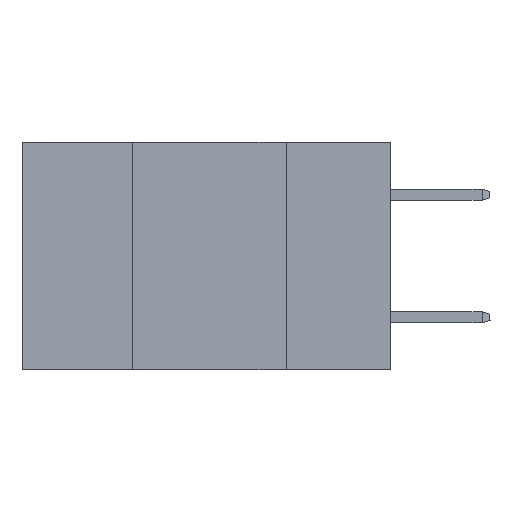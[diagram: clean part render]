
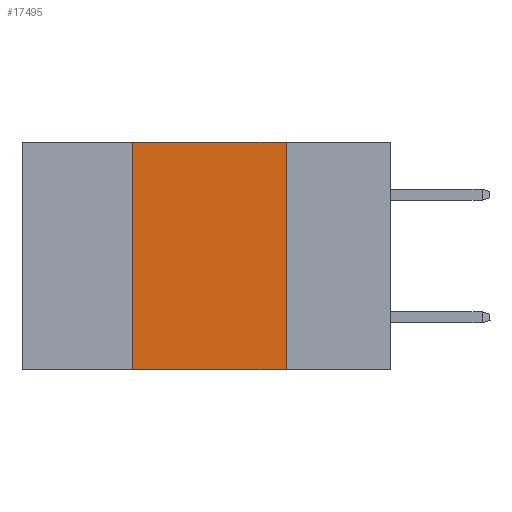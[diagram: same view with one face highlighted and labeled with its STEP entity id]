
A CAD part, left-side view. The second image highlights one B-rep face of the part: STEP entity #17495.
In plain terms, the highlighted planar face has unit normal (-1, 0, 0).
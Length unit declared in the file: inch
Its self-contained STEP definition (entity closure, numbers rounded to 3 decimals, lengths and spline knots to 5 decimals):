
#1050 = CARTESIAN_POINT ( 'NONE',  ( 0., 0.42, -0.37 ) ) ;
#1290 = CARTESIAN_POINT ( 'NONE',  ( 0., 0.17, 0. ) ) ;
#2728 = CARTESIAN_POINT ( 'NONE',  ( 0., 0.42, 0. ) ) ;
#3080 = EDGE_CURVE ( 'NONE', #3220, #10279, #19477, .T. ) ;
#3220 = VERTEX_POINT ( 'NONE', #1050 ) ;
#3921 = EDGE_LOOP ( 'NONE', ( #8095, #25872, #14075, #19346 ) ) ;
#4853 = PLANE ( 'NONE',  #8682 ) ;
#6683 = EDGE_CURVE ( 'NONE', #3220, #9972, #22991, .T. ) ;
#6812 = DIRECTION ( 'NONE',  ( 0., 0., -1. ) ) ;
#7413 = DIRECTION ( 'NONE',  ( 0., 0., -1. ) ) ;
#7713 = CARTESIAN_POINT ( 'NONE',  ( 0., 0.42, 0. ) ) ;
#8095 = ORIENTED_EDGE ( 'NONE', *, *, #16250, .F. ) ;
#8600 = VECTOR ( 'NONE', #19950, 39.37008 ) ;
#8682 = AXIS2_PLACEMENT_3D ( 'NONE', #10731, #18774, #6812 ) ;
#8838 = VECTOR ( 'NONE', #15581, 39.37008 ) ;
#9725 = EDGE_CURVE ( 'NONE', #9972, #20930, #13957, .T. ) ;
#9972 = VERTEX_POINT ( 'NONE', #2728 ) ;
#10279 = VERTEX_POINT ( 'NONE', #11623 ) ;
#10350 = CARTESIAN_POINT ( 'NONE',  ( 0., 0.17, 0. ) ) ;
#10731 = CARTESIAN_POINT ( 'NONE',  ( 0., 0.6, 0. ) ) ;
#11623 = CARTESIAN_POINT ( 'NONE',  ( 0., 0.17, -0.37 ) ) ;
#11712 = DIRECTION ( 'NONE',  ( 0., 0., 1. ) ) ;
#12384 = VECTOR ( 'NONE', #11712, 39.37008 ) ;
#13957 = LINE ( 'NONE', #17960, #8600 ) ;
#14075 = ORIENTED_EDGE ( 'NONE', *, *, #6683, .F. ) ;
#14969 = CARTESIAN_POINT ( 'NONE',  ( 0., 0.6, -0.37 ) ) ;
#15581 = DIRECTION ( 'NONE',  ( 0., -1., 0. ) ) ;
#16250 = EDGE_CURVE ( 'NONE', #20930, #10279, #21958, .T. ) ;
#16631 = VECTOR ( 'NONE', #7413, 39.37008 ) ;
#17495 = ADVANCED_FACE ( 'NONE', ( #23729 ), #4853, .F. ) ;
#17960 = CARTESIAN_POINT ( 'NONE',  ( 0., 0.6, 0. ) ) ;
#18774 = DIRECTION ( 'NONE',  ( 1., 0., 0. ) ) ;
#19346 = ORIENTED_EDGE ( 'NONE', *, *, #3080, .T. ) ;
#19477 = LINE ( 'NONE', #14969, #8838 ) ;
#19950 = DIRECTION ( 'NONE',  ( 0., -1., 0. ) ) ;
#20930 = VERTEX_POINT ( 'NONE', #10350 ) ;
#21958 = LINE ( 'NONE', #1290, #16631 ) ;
#22991 = LINE ( 'NONE', #7713, #12384 ) ;
#23729 = FACE_OUTER_BOUND ( 'NONE', #3921, .T. ) ;
#25872 = ORIENTED_EDGE ( 'NONE', *, *, #9725, .F. ) ;
